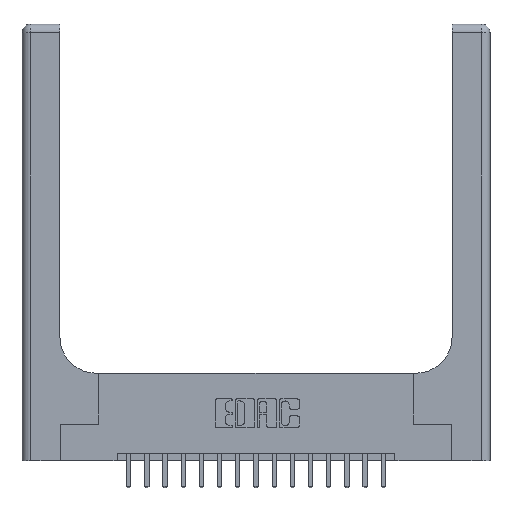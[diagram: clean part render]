
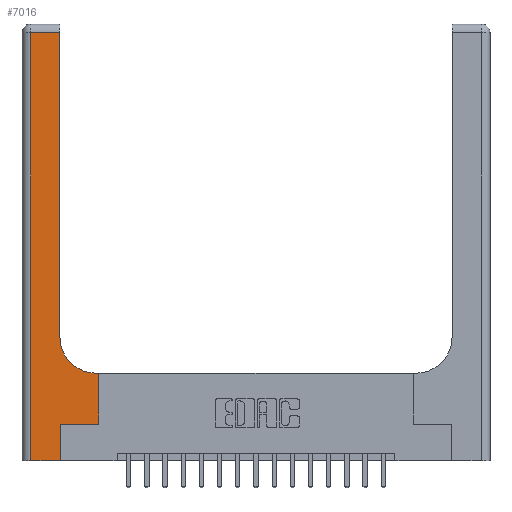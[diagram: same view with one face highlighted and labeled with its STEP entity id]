
A CAD part, top view. The second image highlights one B-rep face of the part: STEP entity #7016.
In plain terms, the highlighted planar face has unit normal (0, 0, 1).
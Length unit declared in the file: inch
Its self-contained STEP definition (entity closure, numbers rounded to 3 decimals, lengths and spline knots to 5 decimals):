
#62 = ORIENTED_EDGE ( 'NONE', *, *, #16715, .T. ) ;
#83 = VERTEX_POINT ( 'NONE', #1826 ) ;
#110 = LINE ( 'NONE', #12143, #3993 ) ;
#126 = ORIENTED_EDGE ( 'NONE', *, *, #17702, .T. ) ;
#593 = ORIENTED_EDGE ( 'NONE', *, *, #16121, .T. ) ;
#1187 = PLANE ( 'NONE',  #8051 ) ;
#1555 = EDGE_LOOP ( 'NONE', ( #3502, #2625, #62, #5556, #593, #18720, #126, #16956, #5131 ) ) ;
#1714 = DIRECTION ( 'NONE',  ( 0., 1., 0. ) ) ;
#1826 = CARTESIAN_POINT ( 'NONE',  ( 0.26, 0.85, 0.37 ) ) ;
#1875 = CARTESIAN_POINT ( 'NONE',  ( 0.51, 0.85, 0.37 ) ) ;
#2625 = ORIENTED_EDGE ( 'NONE', *, *, #5341, .T. ) ;
#2700 = VECTOR ( 'NONE', #3270, 39.37008 ) ;
#2948 = DIRECTION ( 'NONE',  ( 0., 0., -1. ) ) ;
#3270 = DIRECTION ( 'NONE',  ( 1., 0., 0. ) ) ;
#3326 = VERTEX_POINT ( 'NONE', #11656 ) ;
#3489 = CARTESIAN_POINT ( 'NONE',  ( 0.06, 2.94, 0.37 ) ) ;
#3502 = ORIENTED_EDGE ( 'NONE', *, *, #15864, .T. ) ;
#3641 = CARTESIAN_POINT ( 'NONE',  ( 0.528, 0.25, 0.37 ) ) ;
#3993 = VECTOR ( 'NONE', #6348, 39.37008 ) ;
#4005 = CARTESIAN_POINT ( 'NONE',  ( 0., 2.94, 0.37 ) ) ;
#4963 = VERTEX_POINT ( 'NONE', #15636 ) ;
#4984 = LINE ( 'NONE', #5317, #10398 ) ;
#5100 = CARTESIAN_POINT ( 'NONE',  ( 0.265, 0.25, 0.37 ) ) ;
#5131 = ORIENTED_EDGE ( 'NONE', *, *, #13713, .T. ) ;
#5283 = CARTESIAN_POINT ( 'NONE',  ( 0.265, 0., 0.37 ) ) ;
#5317 = CARTESIAN_POINT ( 'NONE',  ( 0.265, 0.25, 0.37 ) ) ;
#5341 = EDGE_CURVE ( 'NONE', #14301, #9890, #18016, .T. ) ;
#5556 = ORIENTED_EDGE ( 'NONE', *, *, #13581, .T. ) ;
#5933 = CARTESIAN_POINT ( 'NONE',  ( 0.26, 2.94, 0.37 ) ) ;
#6072 = DIRECTION ( 'NONE',  ( 0., -1., 0. ) ) ;
#6348 = DIRECTION ( 'NONE',  ( 0., 1., 0. ) ) ;
#6399 = DIRECTION ( 'NONE',  ( 1., 0., 0. ) ) ;
#6510 = CARTESIAN_POINT ( 'NONE',  ( 0.26, 0.6, 0.37 ) ) ;
#6694 = VERTEX_POINT ( 'NONE', #5283 ) ;
#6828 = VECTOR ( 'NONE', #10696, 39.37008 ) ;
#7016 = ADVANCED_FACE ( 'NONE', ( #17069 ), #1187, .F. ) ;
#7435 = CARTESIAN_POINT ( 'NONE',  ( 0.528, 0.25, 0.37 ) ) ;
#7822 = VECTOR ( 'NONE', #6072, 39.37008 ) ;
#8051 = AXIS2_PLACEMENT_3D ( 'NONE', #14612, #2948, #14672 ) ;
#8347 = DIRECTION ( 'NONE',  ( 1., 0., 0. ) ) ;
#8537 = LINE ( 'NONE', #10226, #12602 ) ;
#8606 = LINE ( 'NONE', #14810, #2700 ) ;
#8923 = CARTESIAN_POINT ( 'NONE',  ( 0.06, 3., 0.37 ) ) ;
#9218 = VERTEX_POINT ( 'NONE', #5100 ) ;
#9376 = LINE ( 'NONE', #7435, #17688 ) ;
#9491 = VECTOR ( 'NONE', #17108, 39.37008 ) ;
#9890 = VERTEX_POINT ( 'NONE', #3489 ) ;
#10226 = CARTESIAN_POINT ( 'NONE',  ( 0.26, 3., 0.37 ) ) ;
#10398 = VECTOR ( 'NONE', #8347, 39.37008 ) ;
#10662 = AXIS2_PLACEMENT_3D ( 'NONE', #1875, #12256, #6399 ) ;
#10696 = DIRECTION ( 'NONE',  ( -1., 0., 0. ) ) ;
#11656 = CARTESIAN_POINT ( 'NONE',  ( 0.51, 0.6, 0.37 ) ) ;
#12009 = VERTEX_POINT ( 'NONE', #13780 ) ;
#12143 = CARTESIAN_POINT ( 'NONE',  ( 0.265, 0., 0.37 ) ) ;
#12185 = EDGE_CURVE ( 'NONE', #9218, #15687, #4984, .T. ) ;
#12256 = DIRECTION ( 'NONE',  ( 0., 0., -1. ) ) ;
#12602 = VECTOR ( 'NONE', #18711, 39.37008 ) ;
#12705 = LINE ( 'NONE', #6510, #6828 ) ;
#13258 = EDGE_CURVE ( 'NONE', #4963, #3326, #12705, .T. ) ;
#13581 = EDGE_CURVE ( 'NONE', #12009, #6694, #8606, .T. ) ;
#13713 = EDGE_CURVE ( 'NONE', #3326, #83, #16031, .T. ) ;
#13780 = CARTESIAN_POINT ( 'NONE',  ( 0.06, 0., 0.37 ) ) ;
#14301 = VERTEX_POINT ( 'NONE', #5933 ) ;
#14402 = LINE ( 'NONE', #8923, #7822 ) ;
#14612 = CARTESIAN_POINT ( 'NONE',  ( 0., 3., 0.37 ) ) ;
#14672 = DIRECTION ( 'NONE',  ( -1., 0., 0. ) ) ;
#14810 = CARTESIAN_POINT ( 'NONE',  ( 0., 0., 0.37 ) ) ;
#15636 = CARTESIAN_POINT ( 'NONE',  ( 0.528, 0.6, 0.37 ) ) ;
#15687 = VERTEX_POINT ( 'NONE', #3641 ) ;
#15864 = EDGE_CURVE ( 'NONE', #83, #14301, #8537, .T. ) ;
#16031 = CIRCLE ( 'NONE', #10662, 0.25 ) ;
#16121 = EDGE_CURVE ( 'NONE', #6694, #9218, #110, .T. ) ;
#16715 = EDGE_CURVE ( 'NONE', #9890, #12009, #14402, .T. ) ;
#16956 = ORIENTED_EDGE ( 'NONE', *, *, #13258, .T. ) ;
#17069 = FACE_OUTER_BOUND ( 'NONE', #1555, .T. ) ;
#17108 = DIRECTION ( 'NONE',  ( -1., 0., 0. ) ) ;
#17688 = VECTOR ( 'NONE', #1714, 39.37008 ) ;
#17702 = EDGE_CURVE ( 'NONE', #15687, #4963, #9376, .T. ) ;
#18016 = LINE ( 'NONE', #4005, #9491 ) ;
#18711 = DIRECTION ( 'NONE',  ( 0., 1., 0. ) ) ;
#18720 = ORIENTED_EDGE ( 'NONE', *, *, #12185, .T. ) ;
